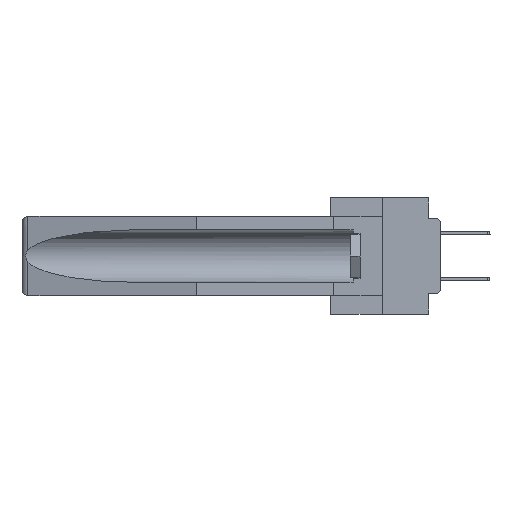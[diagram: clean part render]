
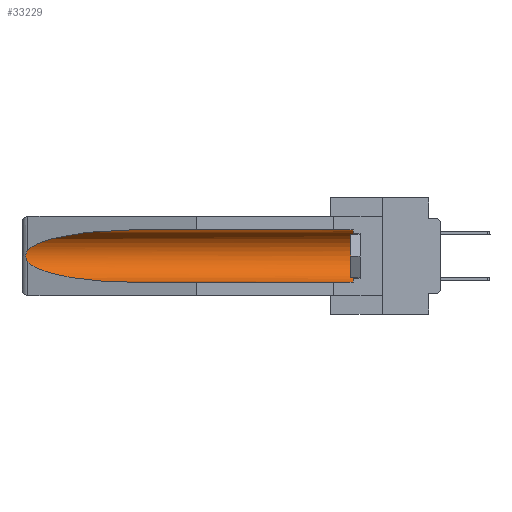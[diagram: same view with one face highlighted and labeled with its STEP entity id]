
A CAD part, left-side view. The second image highlights one B-rep face of the part: STEP entity #33229.
In plain terms, the highlighted cylindrical face has radius 2.857 mm (diameter 5.715 mm), a partial arc.
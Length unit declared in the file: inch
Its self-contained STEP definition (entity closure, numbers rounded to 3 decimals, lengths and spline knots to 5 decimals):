
#162 = CARTESIAN_POINT ( 'NONE',  ( 0.26537, 1.52718, -0.14972 ) ) ;
#2322 = LINE ( 'NONE', #29816, #29785 ) ;
#2354 = EDGE_CURVE ( 'NONE', #11808, #3579, #32071, .T. ) ;
#2645 = EDGE_CURVE ( 'NONE', #22477, #4668, #7403, .T. ) ;
#2720 = CARTESIAN_POINT ( 'NONE',  ( 0.155, 1.07973, -0.059 ) ) ;
#2764 = CARTESIAN_POINT ( 'NONE',  ( 0.26537, 1.52718, -0.14972 ) ) ;
#2886 = CARTESIAN_POINT ( 'NONE',  ( 0.155, 1.07973, -0.059 ) ) ;
#3579 = VERTEX_POINT ( 'NONE', #2764 ) ;
#4190 = AXIS2_PLACEMENT_3D ( 'NONE', #25809, #31295, #28169 ) ;
#4668 = VERTEX_POINT ( 'NONE', #15221 ) ;
#5408 = DIRECTION ( 'NONE',  ( 0., -1., 0. ) ) ;
#5537 = EDGE_CURVE ( 'NONE', #6539, #11808, #2322, .T. ) ;
#5620 = CARTESIAN_POINT ( 'NONE',  ( 0.2673, 1.53269, -0.17917 ) ) ;
#6539 = VERTEX_POINT ( 'NONE', #30949 ) ;
#6701 = CYLINDRICAL_SURFACE ( 'NONE', #4190, 0.1125 ) ;
#6777 = ORIENTED_EDGE ( 'NONE', *, *, #2645, .F. ) ;
#6825 = EDGE_CURVE ( 'NONE', #22477, #6539, #8371, .T. ) ;
#7197 = AXIS2_PLACEMENT_3D ( 'NONE', #30362, #5408, #16162 ) ;
#7403 = LINE ( 'NONE', #18510, #35937 ) ;
#7582 = DIRECTION ( 'NONE',  ( 0., 1., 0. ) ) ;
#8371 = CIRCLE ( 'NONE', #7197, 0.1125 ) ;
#11133 = CARTESIAN_POINT ( 'NONE',  ( 0.155, 1.07973, -0.284 ) ) ;
#11808 = VERTEX_POINT ( 'NONE', #2720 ) ;
#12510 = ORIENTED_EDGE ( 'NONE', *, *, #5537, .T. ) ;
#14417 = EDGE_CURVE ( 'NONE', #3579, #15485, #20904, .T. ) ;
#14599 = CARTESIAN_POINT ( 'NONE',  ( 0.26537, 1.52718, -0.19328 ) ) ;
#14642 = ORIENTED_EDGE ( 'NONE', *, *, #14417, .T. ) ;
#15221 = CARTESIAN_POINT ( 'NONE',  ( 0.155, 1.07973, -0.284 ) ) ;
#15394 = EDGE_CURVE ( 'NONE', #15485, #4668, #27170, .T. ) ;
#15485 = VERTEX_POINT ( 'NONE', #14599 ) ;
#15756 = CARTESIAN_POINT ( 'NONE',  ( 0.21114, 1.30732, -0.284 ) ) ;
#16162 = DIRECTION ( 'NONE',  ( 0., 0., 1. ) ) ;
#18510 = CARTESIAN_POINT ( 'NONE',  ( 0.155, -0.30754, -0.284 ) ) ;
#18933 = CARTESIAN_POINT ( 'NONE',  ( 0.155, 0.126, -0.284 ) ) ;
#19641 = CARTESIAN_POINT ( 'NONE',  ( 0.26597, 1.5296, -0.19026 ) ) ;
#20904 = B_SPLINE_CURVE_WITH_KNOTS ( 'NONE', 3,
 ( #162, #32757, #30037, #30396, #33463, #22018, #5620, #33105, #19641, #24385 ),
 .UNSPECIFIED., .F., .F.,
 ( 4, 2, 2, 2, 4 ),
 ( 0., 0.00029, 0.00058, 0.00087, 0.00117 ),
 .UNSPECIFIED. ) ;
#21436 = DIRECTION ( 'NONE',  ( 0., 1., 0. ) ) ;
#22018 = CARTESIAN_POINT ( 'NONE',  ( 0.2675, 1.53308, -0.17534 ) ) ;
#22177 = CARTESIAN_POINT ( 'NONE',  ( 0.26537, 1.52718, -0.14972 ) ) ;
#22477 = VERTEX_POINT ( 'NONE', #18933 ) ;
#22614 = ORIENTED_EDGE ( 'NONE', *, *, #6825, .T. ) ;
#24366 = CARTESIAN_POINT ( 'NONE',  ( 0.21114, 1.30732, -0.059 ) ) ;
#24385 = CARTESIAN_POINT ( 'NONE',  ( 0.26537, 1.52718, -0.19328 ) ) ;
#25333 = CARTESIAN_POINT ( 'NONE',  ( 0.25451, 1.48313, -0.24835 ) ) ;
#25809 = CARTESIAN_POINT ( 'NONE',  ( 0.155, -0.30754, -0.1715 ) ) ;
#27170 =( BOUNDED_CURVE ( )  B_SPLINE_CURVE ( 3, ( #30989, #25333, #15756, #11133 ),
 .UNSPECIFIED., .F., .F. ) 
 B_SPLINE_CURVE_WITH_KNOTS ( ( 4, 4 ),
 ( 0.1948, 1.5708 ),
 .UNSPECIFIED. ) 
 CURVE ( )  GEOMETRIC_REPRESENTATION_ITEM ( )  RATIONAL_B_SPLINE_CURVE ( ( 1., 0.848, 0.848, 1. ) ) 
 REPRESENTATION_ITEM ( '' )  );
#28169 = DIRECTION ( 'NONE',  ( 0., 0., 1. ) ) ;
#29663 = EDGE_LOOP ( 'NONE', ( #29817, #14642, #32221, #6777, #22614, #12510 ) ) ;
#29785 = VECTOR ( 'NONE', #21436, 39.37008 ) ;
#29816 = CARTESIAN_POINT ( 'NONE',  ( 0.155, -0.30754, -0.059 ) ) ;
#29817 = ORIENTED_EDGE ( 'NONE', *, *, #2354, .T. ) ;
#30037 = CARTESIAN_POINT ( 'NONE',  ( 0.26654, 1.53092, -0.15636 ) ) ;
#30362 = CARTESIAN_POINT ( 'NONE',  ( 0.155, 0.126, -0.1715 ) ) ;
#30396 = CARTESIAN_POINT ( 'NONE',  ( 0.2673, 1.5327, -0.16383 ) ) ;
#30949 = CARTESIAN_POINT ( 'NONE',  ( 0.155, 0.126, -0.059 ) ) ;
#30989 = CARTESIAN_POINT ( 'NONE',  ( 0.26537, 1.52718, -0.19328 ) ) ;
#31295 = DIRECTION ( 'NONE',  ( 0., 1., 0. ) ) ;
#32071 =( BOUNDED_CURVE ( )  B_SPLINE_CURVE ( 3, ( #2886, #24366, #32740, #22177 ),
 .UNSPECIFIED., .F., .F. ) 
 B_SPLINE_CURVE_WITH_KNOTS ( ( 4, 4 ),
 ( 4.71239, 6.08839 ),
 .UNSPECIFIED. ) 
 CURVE ( )  GEOMETRIC_REPRESENTATION_ITEM ( )  RATIONAL_B_SPLINE_CURVE ( ( 1., 0.848, 0.848, 1. ) ) 
 REPRESENTATION_ITEM ( '' )  );
#32221 = ORIENTED_EDGE ( 'NONE', *, *, #15394, .T. ) ;
#32740 = CARTESIAN_POINT ( 'NONE',  ( 0.25451, 1.48313, -0.09465 ) ) ;
#32757 = CARTESIAN_POINT ( 'NONE',  ( 0.26597, 1.52961, -0.15275 ) ) ;
#33105 = CARTESIAN_POINT ( 'NONE',  ( 0.26655, 1.53094, -0.18657 ) ) ;
#33229 = ADVANCED_FACE ( 'NONE', ( #33991 ), #6701, .F. ) ;
#33463 = CARTESIAN_POINT ( 'NONE',  ( 0.2675, 1.53308, -0.16763 ) ) ;
#33991 = FACE_OUTER_BOUND ( 'NONE', #29663, .T. ) ;
#35937 = VECTOR ( 'NONE', #7582, 39.37008 ) ;
